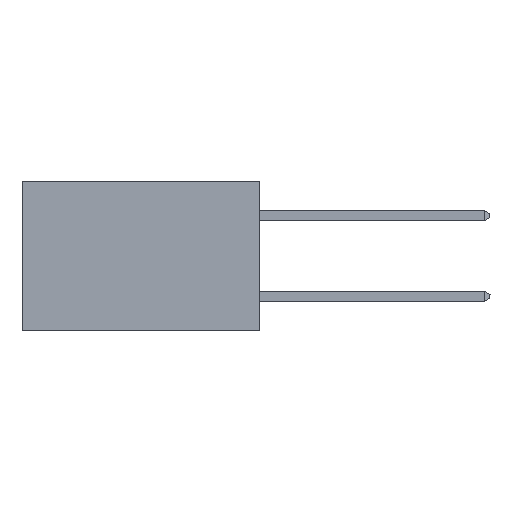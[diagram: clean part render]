
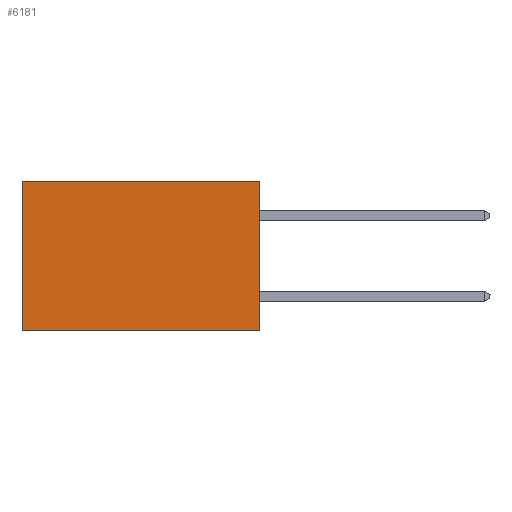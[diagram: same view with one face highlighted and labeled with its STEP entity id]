
A CAD part, left-side view. The second image highlights one B-rep face of the part: STEP entity #6181.
In plain terms, the highlighted planar face has unit normal (-1, 0, 0).
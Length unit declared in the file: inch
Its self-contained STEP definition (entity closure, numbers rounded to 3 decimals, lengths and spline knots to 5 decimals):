
#776 = ORIENTED_EDGE ( 'NONE', *, *, #5261, .F. ) ;
#1627 = CARTESIAN_POINT ( 'NONE',  ( 0.277, 0., -0.37 ) ) ;
#1681 = VERTEX_POINT ( 'NONE', #4064 ) ;
#1784 = VERTEX_POINT ( 'NONE', #3566 ) ;
#3011 = CARTESIAN_POINT ( 'NONE',  ( 0.277, 0.59, -0.37 ) ) ;
#3202 = LINE ( 'NONE', #6305, #25083 ) ;
#3566 = CARTESIAN_POINT ( 'NONE',  ( 0.277, 0., -0.37 ) ) ;
#3748 = DIRECTION ( 'NONE',  ( 0., 0., -1. ) ) ;
#3803 = LINE ( 'NONE', #6578, #14281 ) ;
#3896 = ORIENTED_EDGE ( 'NONE', *, *, #19606, .T. ) ;
#4064 = CARTESIAN_POINT ( 'NONE',  ( 0.277, 0., 0. ) ) ;
#4258 = CARTESIAN_POINT ( 'NONE',  ( 0.277, 0.59, -0.37 ) ) ;
#4727 = CARTESIAN_POINT ( 'NONE',  ( 0.277, 0.59, 0. ) ) ;
#5261 = EDGE_CURVE ( 'NONE', #1784, #9323, #24230, .T. ) ;
#6181 = ADVANCED_FACE ( 'NONE', ( #19336 ), #14177, .F. ) ;
#6305 = CARTESIAN_POINT ( 'NONE',  ( 0.277, 0., -0.37 ) ) ;
#6394 = DIRECTION ( 'NONE',  ( 0., 0., -1. ) ) ;
#6578 = CARTESIAN_POINT ( 'NONE',  ( 0.277, 0., 0. ) ) ;
#7360 = LINE ( 'NONE', #4258, #17681 ) ;
#7806 = VERTEX_POINT ( 'NONE', #4727 ) ;
#8658 = DIRECTION ( 'NONE',  ( 0., 1., 0. ) ) ;
#9323 = VERTEX_POINT ( 'NONE', #3011 ) ;
#13859 = EDGE_CURVE ( 'NONE', #7806, #9323, #7360, .T. ) ;
#14177 = PLANE ( 'NONE',  #21563 ) ;
#14281 = VECTOR ( 'NONE', #8658, 39.37008 ) ;
#15991 = ORIENTED_EDGE ( 'NONE', *, *, #13859, .T. ) ;
#16174 = ORIENTED_EDGE ( 'NONE', *, *, #17800, .F. ) ;
#16222 = DIRECTION ( 'NONE',  ( 1., 0., 0. ) ) ;
#17681 = VECTOR ( 'NONE', #6394, 39.37008 ) ;
#17800 = EDGE_CURVE ( 'NONE', #1681, #1784, #3202, .T. ) ;
#18090 = DIRECTION ( 'NONE',  ( 0., 1., 0. ) ) ;
#18412 = CARTESIAN_POINT ( 'NONE',  ( 0.277, 0., -0.37 ) ) ;
#19336 = FACE_OUTER_BOUND ( 'NONE', #24831, .T. ) ;
#19493 = VECTOR ( 'NONE', #18090, 39.37008 ) ;
#19606 = EDGE_CURVE ( 'NONE', #1681, #7806, #3803, .T. ) ;
#20682 = DIRECTION ( 'NONE',  ( 0., 0., -1. ) ) ;
#21563 = AXIS2_PLACEMENT_3D ( 'NONE', #1627, #16222, #3748 ) ;
#24230 = LINE ( 'NONE', #18412, #19493 ) ;
#24831 = EDGE_LOOP ( 'NONE', ( #15991, #776, #16174, #3896 ) ) ;
#25083 = VECTOR ( 'NONE', #20682, 39.37008 ) ;
